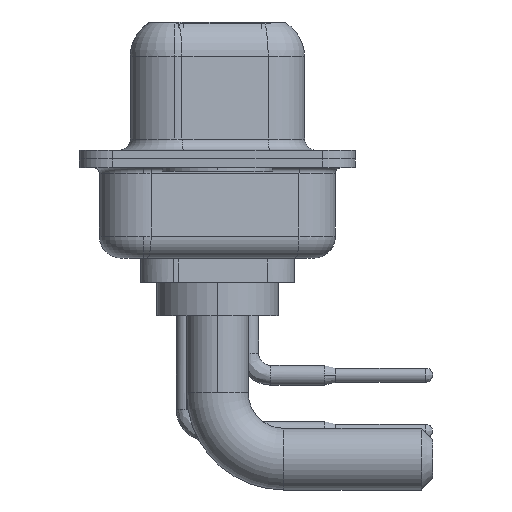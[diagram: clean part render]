
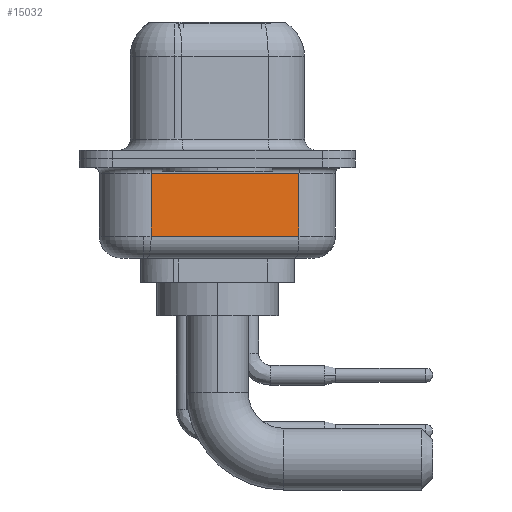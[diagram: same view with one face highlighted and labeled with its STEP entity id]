
A CAD part, left-side view. The second image highlights one B-rep face of the part: STEP entity #15032.
In plain terms, the highlighted planar face has unit normal (-0.985, -0.174, 0).
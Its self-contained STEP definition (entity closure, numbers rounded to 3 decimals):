
#1035 = CARTESIAN_POINT ( 'NONE',  ( 4.062, -3.697, -0.65 ) ) ;
#1512 = CARTESIAN_POINT ( 'NONE',  ( 2.88, 3.003, -0.65 ) ) ;
#1901 = DIRECTION ( 'NONE',  ( 0.174, -0.985, 0. ) ) ;
#3024 = CARTESIAN_POINT ( 'NONE',  ( 2.88, 3.003, -4.5 ) ) ;
#4081 = EDGE_CURVE ( 'NONE', #11876, #13318, #6210, .T. ) ;
#4149 = DIRECTION ( 'NONE',  ( -0.174, 0.985, 0. ) ) ;
#5350 = CARTESIAN_POINT ( 'NONE',  ( 2.88, 3.003, -3.5 ) ) ;
#5366 = FACE_OUTER_BOUND ( 'NONE', #12489, .T. ) ;
#5566 = PLANE ( 'NONE',  #13228 ) ;
#5669 = EDGE_CURVE ( 'NONE', #15398, #9609, #16907, .T. ) ;
#5840 = DIRECTION ( 'NONE',  ( 0., 0., 1. ) ) ;
#6032 = VECTOR ( 'NONE', #18388, 1000. ) ;
#6210 = LINE ( 'NONE', #8717, #17107 ) ;
#7259 = DIRECTION ( 'NONE',  ( 0., 0., 1. ) ) ;
#7522 = CARTESIAN_POINT ( 'NONE',  ( 4.062, -3.697, -4.5 ) ) ;
#8081 = VECTOR ( 'NONE', #7259, 1000. ) ;
#8717 = CARTESIAN_POINT ( 'NONE',  ( 2.88, 3.003, -3.5 ) ) ;
#9172 = ORIENTED_EDGE ( 'NONE', *, *, #4081, .T. ) ;
#9609 = VERTEX_POINT ( 'NONE', #10607 ) ;
#9937 = CARTESIAN_POINT ( 'NONE',  ( 4.062, -3.697, -3.5 ) ) ;
#10607 = CARTESIAN_POINT ( 'NONE',  ( 2.88, 3.003, -0.65 ) ) ;
#10640 = ORIENTED_EDGE ( 'NONE', *, *, #5669, .T. ) ;
#11029 = EDGE_CURVE ( 'NONE', #13318, #15398, #11787, .T. ) ;
#11591 = EDGE_CURVE ( 'NONE', #11876, #9609, #11769, .T. ) ;
#11769 = LINE ( 'NONE', #3024, #16427 ) ;
#11787 = LINE ( 'NONE', #7522, #8081 ) ;
#11876 = VERTEX_POINT ( 'NONE', #5350 ) ;
#12489 = EDGE_LOOP ( 'NONE', ( #12897, #9172, #16645, #10640 ) ) ;
#12897 = ORIENTED_EDGE ( 'NONE', *, *, #11591, .F. ) ;
#13228 = AXIS2_PLACEMENT_3D ( 'NONE', #16915, #15326, #4149 ) ;
#13318 = VERTEX_POINT ( 'NONE', #9937 ) ;
#15032 = ADVANCED_FACE ( 'NONE', ( #5366 ), #5566, .F. ) ;
#15326 = DIRECTION ( 'NONE',  ( 0.985, 0.174, 0. ) ) ;
#15398 = VERTEX_POINT ( 'NONE', #1035 ) ;
#16427 = VECTOR ( 'NONE', #5840, 1000. ) ;
#16645 = ORIENTED_EDGE ( 'NONE', *, *, #11029, .T. ) ;
#16907 = LINE ( 'NONE', #1512, #6032 ) ;
#16915 = CARTESIAN_POINT ( 'NONE',  ( 2.88, 3.003, -4.5 ) ) ;
#17107 = VECTOR ( 'NONE', #1901, 1000. ) ;
#18388 = DIRECTION ( 'NONE',  ( -0.174, 0.985, 0. ) ) ;
